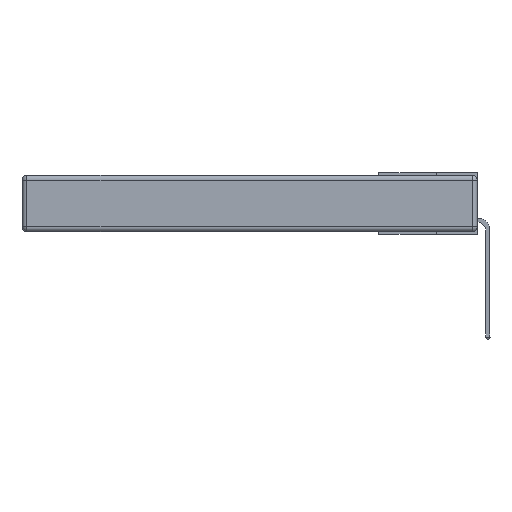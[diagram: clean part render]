
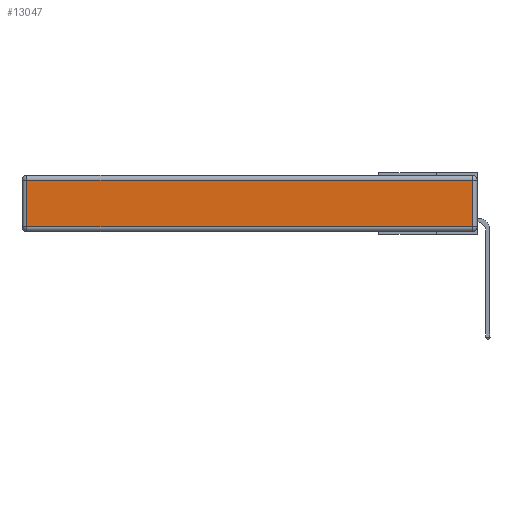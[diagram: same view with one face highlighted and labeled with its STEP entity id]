
A CAD part, left-side view. The second image highlights one B-rep face of the part: STEP entity #13047.
In plain terms, the highlighted planar face has unit normal (-1, 0, 0).
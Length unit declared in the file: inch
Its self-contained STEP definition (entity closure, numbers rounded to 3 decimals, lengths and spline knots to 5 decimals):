
#1779 = VECTOR ( 'NONE', #13804, 39.37008 ) ;
#1825 = VERTEX_POINT ( 'NONE', #11855 ) ;
#2184 = FACE_OUTER_BOUND ( 'NONE', #21338, .T. ) ;
#3231 = VERTEX_POINT ( 'NONE', #13162 ) ;
#4263 = DIRECTION ( 'NONE',  ( -1., 0., 0. ) ) ;
#4570 = ORIENTED_EDGE ( 'NONE', *, *, #18909, .T. ) ;
#4816 = LINE ( 'NONE', #21504, #12405 ) ;
#5694 = ORIENTED_EDGE ( 'NONE', *, *, #17589, .T. ) ;
#6500 = LINE ( 'NONE', #20792, #31064 ) ;
#6618 = ORIENTED_EDGE ( 'NONE', *, *, #27541, .T. ) ;
#6783 = DIRECTION ( 'NONE',  ( 0., -1., 0. ) ) ;
#8050 = DIRECTION ( 'NONE',  ( 0., 1., 0. ) ) ;
#11215 = EDGE_CURVE ( 'NONE', #21554, #19431, #4816, .T. ) ;
#11389 = CARTESIAN_POINT ( 'NONE',  ( 0., 0., -0.343 ) ) ;
#11774 = VECTOR ( 'NONE', #16957, 39.37008 ) ;
#11855 = CARTESIAN_POINT ( 'NONE',  ( 0., 0.03, -0.03 ) ) ;
#11946 = CARTESIAN_POINT ( 'NONE',  ( 0., 2.72, -0.313 ) ) ;
#12405 = VECTOR ( 'NONE', #6783, 39.37008 ) ;
#13047 = ADVANCED_FACE ( 'NONE', ( #2184 ), #14177, .T. ) ;
#13162 = CARTESIAN_POINT ( 'NONE',  ( 0., 2.72, -0.03 ) ) ;
#13804 = DIRECTION ( 'NONE',  ( 0., 0., 1. ) ) ;
#14177 = PLANE ( 'NONE',  #20563 ) ;
#14922 = ORIENTED_EDGE ( 'NONE', *, *, #11215, .T. ) ;
#16072 = LINE ( 'NONE', #31477, #1779 ) ;
#16696 = DIRECTION ( 'NONE',  ( 0., 0., 1. ) ) ;
#16957 = DIRECTION ( 'NONE',  ( 0., 0., -1. ) ) ;
#17589 = EDGE_CURVE ( 'NONE', #3231, #21554, #23640, .T. ) ;
#18909 = EDGE_CURVE ( 'NONE', #19431, #1825, #16072, .T. ) ;
#19431 = VERTEX_POINT ( 'NONE', #31227 ) ;
#20563 = AXIS2_PLACEMENT_3D ( 'NONE', #11389, #4263, #16696 ) ;
#20792 = CARTESIAN_POINT ( 'NONE',  ( 0., 2.75, -0.03 ) ) ;
#21338 = EDGE_LOOP ( 'NONE', ( #14922, #4570, #6618, #5694 ) ) ;
#21504 = CARTESIAN_POINT ( 'NONE',  ( 0., 0., -0.313 ) ) ;
#21554 = VERTEX_POINT ( 'NONE', #11946 ) ;
#23640 = LINE ( 'NONE', #29364, #11774 ) ;
#27541 = EDGE_CURVE ( 'NONE', #1825, #3231, #6500, .T. ) ;
#29364 = CARTESIAN_POINT ( 'NONE',  ( 0., 2.72, -0.343 ) ) ;
#31064 = VECTOR ( 'NONE', #8050, 39.37008 ) ;
#31227 = CARTESIAN_POINT ( 'NONE',  ( 0., 0.03, -0.313 ) ) ;
#31477 = CARTESIAN_POINT ( 'NONE',  ( 0., 0.03, -0.343 ) ) ;
